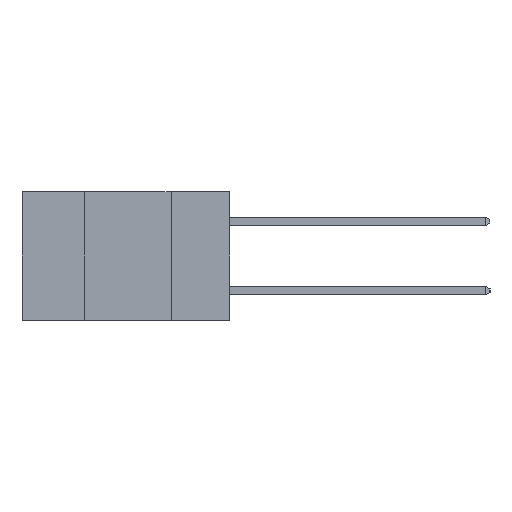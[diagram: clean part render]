
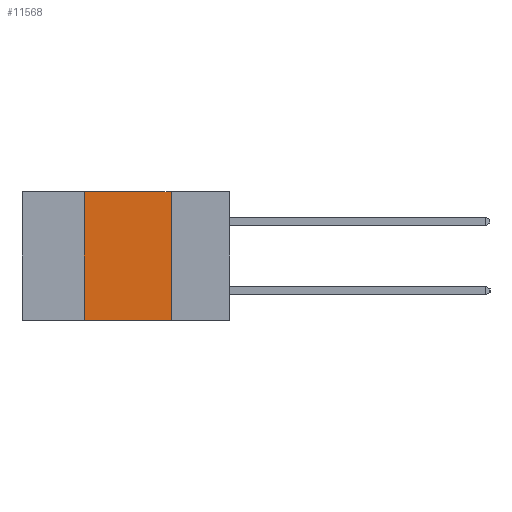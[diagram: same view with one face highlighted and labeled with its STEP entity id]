
A CAD part, left-side view. The second image highlights one B-rep face of the part: STEP entity #11568.
In plain terms, the highlighted planar face has unit normal (-1, 0, 0).
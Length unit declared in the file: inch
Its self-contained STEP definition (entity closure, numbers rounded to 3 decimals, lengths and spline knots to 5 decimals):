
#772 = CARTESIAN_POINT ( 'NONE',  ( 0., 0.6, 0. ) ) ;
#998 = EDGE_CURVE ( 'NONE', #9544, #6491, #7229, .T. ) ;
#1129 = VERTEX_POINT ( 'NONE', #2726 ) ;
#1715 = EDGE_CURVE ( 'NONE', #6491, #12904, #6866, .T. ) ;
#1719 = LINE ( 'NONE', #8334, #12342 ) ;
#2150 = ORIENTED_EDGE ( 'NONE', *, *, #11649, .T. ) ;
#2726 = CARTESIAN_POINT ( 'NONE',  ( 0., 0.42, -0.37 ) ) ;
#3754 = CARTESIAN_POINT ( 'NONE',  ( 0., 0.42, -0.37 ) ) ;
#3818 = DIRECTION ( 'NONE',  ( 0., 0., 1. ) ) ;
#4682 = CARTESIAN_POINT ( 'NONE',  ( 0., 0.42, 0. ) ) ;
#4908 = VECTOR ( 'NONE', #3818, 39.37008 ) ;
#5093 = FACE_OUTER_BOUND ( 'NONE', #7744, .T. ) ;
#6022 = CARTESIAN_POINT ( 'NONE',  ( 0., 0.17, -0.37 ) ) ;
#6491 = VERTEX_POINT ( 'NONE', #6930 ) ;
#6520 = VECTOR ( 'NONE', #7200, 39.37008 ) ;
#6866 = LINE ( 'NONE', #6891, #6520 ) ;
#6891 = CARTESIAN_POINT ( 'NONE',  ( 0., 0.17, -0.37 ) ) ;
#6930 = CARTESIAN_POINT ( 'NONE',  ( 0., 0.17, 0. ) ) ;
#7200 = DIRECTION ( 'NONE',  ( 0., 0., -1. ) ) ;
#7229 = LINE ( 'NONE', #772, #12644 ) ;
#7744 = EDGE_LOOP ( 'NONE', ( #9304, #11071, #12125, #2150 ) ) ;
#8334 = CARTESIAN_POINT ( 'NONE',  ( 0., 0.6, -0.37 ) ) ;
#8341 = DIRECTION ( 'NONE',  ( 0., -1., 0. ) ) ;
#8735 = DIRECTION ( 'NONE',  ( 0., 0., -1. ) ) ;
#8752 = DIRECTION ( 'NONE',  ( 1., 0., 0. ) ) ;
#8770 = PLANE ( 'NONE',  #11934 ) ;
#8813 = CARTESIAN_POINT ( 'NONE',  ( 0., 0.6, 0. ) ) ;
#9304 = ORIENTED_EDGE ( 'NONE', *, *, #1715, .F. ) ;
#9544 = VERTEX_POINT ( 'NONE', #4682 ) ;
#11071 = ORIENTED_EDGE ( 'NONE', *, *, #998, .F. ) ;
#11568 = ADVANCED_FACE ( 'NONE', ( #5093 ), #8770, .F. ) ;
#11649 = EDGE_CURVE ( 'NONE', #1129, #12904, #1719, .T. ) ;
#11658 = DIRECTION ( 'NONE',  ( 0., -1., 0. ) ) ;
#11934 = AXIS2_PLACEMENT_3D ( 'NONE', #8813, #8752, #8735 ) ;
#12125 = ORIENTED_EDGE ( 'NONE', *, *, #12309, .F. ) ;
#12309 = EDGE_CURVE ( 'NONE', #1129, #9544, #13108, .T. ) ;
#12342 = VECTOR ( 'NONE', #8341, 39.37008 ) ;
#12644 = VECTOR ( 'NONE', #11658, 39.37008 ) ;
#12904 = VERTEX_POINT ( 'NONE', #6022 ) ;
#13108 = LINE ( 'NONE', #3754, #4908 ) ;
